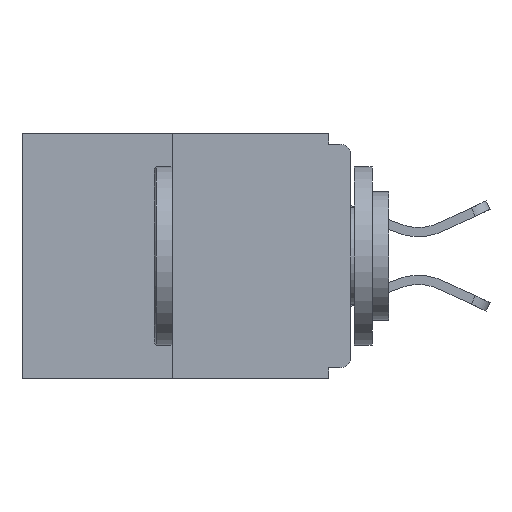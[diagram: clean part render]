
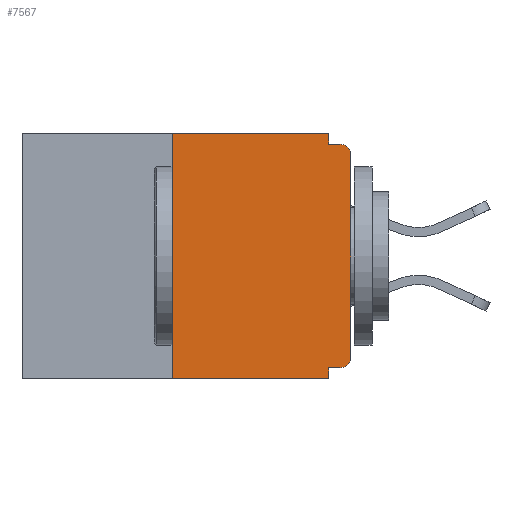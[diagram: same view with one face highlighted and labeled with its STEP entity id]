
A CAD part, left-side view. The second image highlights one B-rep face of the part: STEP entity #7567.
In plain terms, the highlighted planar face has unit normal (-1, 0, 0).
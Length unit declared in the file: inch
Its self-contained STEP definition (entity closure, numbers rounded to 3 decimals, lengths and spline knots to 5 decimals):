
#162 = VECTOR ( 'NONE', #18164, 39.37008 ) ;
#189 = EDGE_CURVE ( 'NONE', #4534, #6159, #8914, .T. ) ;
#232 = VERTEX_POINT ( 'NONE', #12768 ) ;
#702 = ORIENTED_EDGE ( 'NONE', *, *, #189, .T. ) ;
#814 = LINE ( 'NONE', #15116, #15864 ) ;
#1184 = EDGE_CURVE ( 'NONE', #5728, #4234, #4760, .T. ) ;
#1272 = AXIS2_PLACEMENT_3D ( 'NONE', #18843, #10036, #2991 ) ;
#2144 = CARTESIAN_POINT ( 'NONE',  ( 0., 0., 0. ) ) ;
#2234 = CIRCLE ( 'NONE', #1272, 0.015 ) ;
#2991 = DIRECTION ( 'NONE',  ( 0., 0., -1. ) ) ;
#3806 = CARTESIAN_POINT ( 'NONE',  ( 0., 0.031, -0.343 ) ) ;
#4234 = VERTEX_POINT ( 'NONE', #14007 ) ;
#4471 = LINE ( 'NONE', #18100, #162 ) ;
#4508 = ORIENTED_EDGE ( 'NONE', *, *, #16105, .F. ) ;
#4534 = VERTEX_POINT ( 'NONE', #8165 ) ;
#4760 = CIRCLE ( 'NONE', #6821, 0.015 ) ;
#5021 = VECTOR ( 'NONE', #12653, 39.37008 ) ;
#5031 = LINE ( 'NONE', #14213, #14178 ) ;
#5036 = DIRECTION ( 'NONE',  ( 0., 0., -1. ) ) ;
#5447 = DIRECTION ( 'NONE',  ( 0., 0., 1. ) ) ;
#5728 = VERTEX_POINT ( 'NONE', #8329 ) ;
#6159 = VERTEX_POINT ( 'NONE', #7540 ) ;
#6344 = VECTOR ( 'NONE', #7325, 39.37008 ) ;
#6496 = CARTESIAN_POINT ( 'NONE',  ( 0., 0.015, -0.313 ) ) ;
#6695 = LINE ( 'NONE', #2144, #13787 ) ;
#6821 = AXIS2_PLACEMENT_3D ( 'NONE', #6496, #8044, #10997 ) ;
#7297 = EDGE_CURVE ( 'NONE', #5728, #232, #814, .T. ) ;
#7325 = DIRECTION ( 'NONE',  ( 0., 0., -1. ) ) ;
#7540 = CARTESIAN_POINT ( 'NONE',  ( 0., 0.031, -0.343 ) ) ;
#7567 = ADVANCED_FACE ( 'NONE', ( #14941 ), #18866, .F. ) ;
#7644 = ORIENTED_EDGE ( 'NONE', *, *, #10978, .F. ) ;
#7763 = ORIENTED_EDGE ( 'NONE', *, *, #16741, .T. ) ;
#7896 = ORIENTED_EDGE ( 'NONE', *, *, #16515, .F. ) ;
#7915 = VERTEX_POINT ( 'NONE', #16919 ) ;
#8044 = DIRECTION ( 'NONE',  ( -1., 0., 0. ) ) ;
#8165 = CARTESIAN_POINT ( 'NONE',  ( 0., 0.25, -0.343 ) ) ;
#8307 = EDGE_CURVE ( 'NONE', #4234, #17796, #6695, .T. ) ;
#8329 = CARTESIAN_POINT ( 'NONE',  ( 0., 0.015, -0.328 ) ) ;
#8914 = LINE ( 'NONE', #9713, #5021 ) ;
#8939 = VERTEX_POINT ( 'NONE', #16822 ) ;
#9103 = VECTOR ( 'NONE', #12190, 39.37008 ) ;
#9168 = VERTEX_POINT ( 'NONE', #10573 ) ;
#9341 = DIRECTION ( 'NONE',  ( 0., 1., 0. ) ) ;
#9626 = EDGE_CURVE ( 'NONE', #4534, #8939, #5031, .T. ) ;
#9713 = CARTESIAN_POINT ( 'NONE',  ( 0., 0.46, -0.343 ) ) ;
#9798 = LINE ( 'NONE', #3806, #16166 ) ;
#10036 = DIRECTION ( 'NONE',  ( -1., 0., 0. ) ) ;
#10063 = DIRECTION ( 'NONE',  ( 0., 0., -1. ) ) ;
#10573 = CARTESIAN_POINT ( 'NONE',  ( 0., 0.031, 0. ) ) ;
#10978 = EDGE_CURVE ( 'NONE', #9168, #7915, #12101, .T. ) ;
#10997 = DIRECTION ( 'NONE',  ( 0., 0., -1. ) ) ;
#11008 = CARTESIAN_POINT ( 'NONE',  ( 0., 0., -0.03 ) ) ;
#11456 = VERTEX_POINT ( 'NONE', #11480 ) ;
#11480 = CARTESIAN_POINT ( 'NONE',  ( 0., 0.015, -0.015 ) ) ;
#11676 = AXIS2_PLACEMENT_3D ( 'NONE', #15975, #17314, #10063 ) ;
#12101 = LINE ( 'NONE', #12228, #6344 ) ;
#12188 = ORIENTED_EDGE ( 'NONE', *, *, #17413, .F. ) ;
#12190 = DIRECTION ( 'NONE',  ( 0., -1., 0. ) ) ;
#12228 = CARTESIAN_POINT ( 'NONE',  ( 0., 0.031, 0. ) ) ;
#12375 = DIRECTION ( 'NONE',  ( 0., 0., 1. ) ) ;
#12383 = CARTESIAN_POINT ( 'NONE',  ( 0., 0.46, 0. ) ) ;
#12618 = ORIENTED_EDGE ( 'NONE', *, *, #9626, .F. ) ;
#12653 = DIRECTION ( 'NONE',  ( 0., -1., 0. ) ) ;
#12768 = CARTESIAN_POINT ( 'NONE',  ( 0., 0.031, -0.328 ) ) ;
#13744 = ORIENTED_EDGE ( 'NONE', *, *, #8307, .T. ) ;
#13787 = VECTOR ( 'NONE', #12375, 39.37008 ) ;
#14007 = CARTESIAN_POINT ( 'NONE',  ( 0., 0., -0.313 ) ) ;
#14178 = VECTOR ( 'NONE', #5447, 39.37008 ) ;
#14213 = CARTESIAN_POINT ( 'NONE',  ( 0., 0.25, 0. ) ) ;
#14941 = FACE_OUTER_BOUND ( 'NONE', #18006, .T. ) ;
#15116 = CARTESIAN_POINT ( 'NONE',  ( 0., 0., -0.328 ) ) ;
#15437 = ORIENTED_EDGE ( 'NONE', *, *, #7297, .F. ) ;
#15864 = VECTOR ( 'NONE', #9341, 39.37008 ) ;
#15975 = CARTESIAN_POINT ( 'NONE',  ( 0., 0.46, 0. ) ) ;
#16105 = EDGE_CURVE ( 'NONE', #232, #6159, #9798, .T. ) ;
#16166 = VECTOR ( 'NONE', #5036, 39.37008 ) ;
#16515 = EDGE_CURVE ( 'NONE', #8939, #9168, #17753, .T. ) ;
#16741 = EDGE_CURVE ( 'NONE', #17796, #11456, #2234, .T. ) ;
#16822 = CARTESIAN_POINT ( 'NONE',  ( 0., 0.25, 0. ) ) ;
#16919 = CARTESIAN_POINT ( 'NONE',  ( 0., 0.031, -0.015 ) ) ;
#17314 = DIRECTION ( 'NONE',  ( 1., 0., 0. ) ) ;
#17323 = ORIENTED_EDGE ( 'NONE', *, *, #1184, .T. ) ;
#17413 = EDGE_CURVE ( 'NONE', #7915, #11456, #4471, .T. ) ;
#17753 = LINE ( 'NONE', #12383, #9103 ) ;
#17796 = VERTEX_POINT ( 'NONE', #11008 ) ;
#18006 = EDGE_LOOP ( 'NONE', ( #7896, #12618, #702, #4508, #15437, #17323, #13744, #7763, #12188, #7644 ) ) ;
#18100 = CARTESIAN_POINT ( 'NONE',  ( 0., 0., -0.015 ) ) ;
#18164 = DIRECTION ( 'NONE',  ( 0., -1., 0. ) ) ;
#18843 = CARTESIAN_POINT ( 'NONE',  ( 0., 0.015, -0.03 ) ) ;
#18866 = PLANE ( 'NONE',  #11676 ) ;
